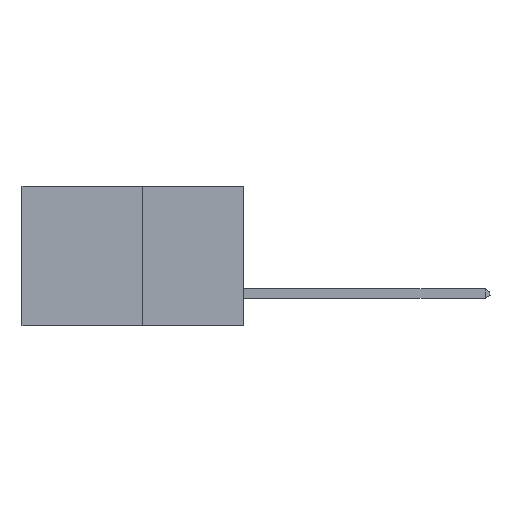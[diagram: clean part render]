
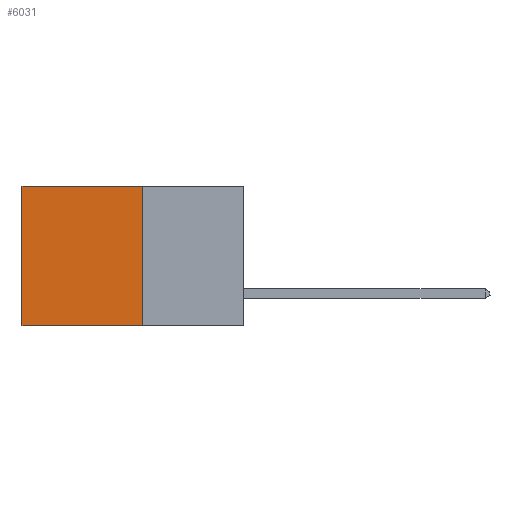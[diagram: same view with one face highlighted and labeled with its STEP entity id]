
A CAD part, left-side view. The second image highlights one B-rep face of the part: STEP entity #6031.
In plain terms, the highlighted planar face has unit normal (-1, 0, 0).
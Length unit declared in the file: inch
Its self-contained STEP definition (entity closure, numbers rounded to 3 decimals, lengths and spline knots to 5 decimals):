
#248 = EDGE_CURVE ( 'NONE', #10938, #4359, #6417, .T. ) ;
#1336 = DIRECTION ( 'NONE',  ( 1., 0., 0. ) ) ;
#1435 = EDGE_CURVE ( 'NONE', #12349, #2503, #1498, .T. ) ;
#1498 = LINE ( 'NONE', #10430, #12309 ) ;
#1690 = EDGE_CURVE ( 'NONE', #12349, #10938, #6663, .T. ) ;
#2080 = DIRECTION ( 'NONE',  ( 0., 0., -1. ) ) ;
#2503 = VERTEX_POINT ( 'NONE', #3233 ) ;
#2925 = CARTESIAN_POINT ( 'NONE',  ( 0.277, 0.27, -0.37 ) ) ;
#3233 = CARTESIAN_POINT ( 'NONE',  ( 0.277, 0.59, 0. ) ) ;
#3308 = ORIENTED_EDGE ( 'NONE', *, *, #7790, .T. ) ;
#3382 = ORIENTED_EDGE ( 'NONE', *, *, #248, .F. ) ;
#3387 = CARTESIAN_POINT ( 'NONE',  ( 0.277, 0.27, -0.37 ) ) ;
#3745 = FACE_OUTER_BOUND ( 'NONE', #6903, .T. ) ;
#3776 = ORIENTED_EDGE ( 'NONE', *, *, #1690, .F. ) ;
#4134 = ORIENTED_EDGE ( 'NONE', *, *, #1435, .T. ) ;
#4359 = VERTEX_POINT ( 'NONE', #7777 ) ;
#4891 = CARTESIAN_POINT ( 'NONE',  ( 0.277, 0.27, -0.37 ) ) ;
#5685 = PLANE ( 'NONE',  #12812 ) ;
#6031 = ADVANCED_FACE ( 'NONE', ( #3745 ), #5685, .F. ) ;
#6400 = LINE ( 'NONE', #10934, #11286 ) ;
#6417 = LINE ( 'NONE', #4891, #11306 ) ;
#6663 = LINE ( 'NONE', #3387, #9011 ) ;
#6903 = EDGE_LOOP ( 'NONE', ( #3308, #3382, #3776, #4134 ) ) ;
#7453 = DIRECTION ( 'NONE',  ( 0., 1., 0. ) ) ;
#7680 = CARTESIAN_POINT ( 'NONE',  ( 0.277, 0.27, -0.37 ) ) ;
#7777 = CARTESIAN_POINT ( 'NONE',  ( 0.277, 0.59, -0.37 ) ) ;
#7790 = EDGE_CURVE ( 'NONE', #2503, #4359, #6400, .T. ) ;
#8691 = DIRECTION ( 'NONE',  ( 0., 0., -1. ) ) ;
#9011 = VECTOR ( 'NONE', #2080, 39.37008 ) ;
#9992 = DIRECTION ( 'NONE',  ( 0., 0., -1. ) ) ;
#10430 = CARTESIAN_POINT ( 'NONE',  ( 0.277, 0.27, 0. ) ) ;
#10873 = DIRECTION ( 'NONE',  ( 0., 1., 0. ) ) ;
#10934 = CARTESIAN_POINT ( 'NONE',  ( 0.277, 0.59, -0.37 ) ) ;
#10938 = VERTEX_POINT ( 'NONE', #2925 ) ;
#11286 = VECTOR ( 'NONE', #9992, 39.37008 ) ;
#11306 = VECTOR ( 'NONE', #10873, 39.37008 ) ;
#12309 = VECTOR ( 'NONE', #7453, 39.37008 ) ;
#12349 = VERTEX_POINT ( 'NONE', #12659 ) ;
#12659 = CARTESIAN_POINT ( 'NONE',  ( 0.277, 0.27, 0. ) ) ;
#12812 = AXIS2_PLACEMENT_3D ( 'NONE', #7680, #1336, #8691 ) ;
